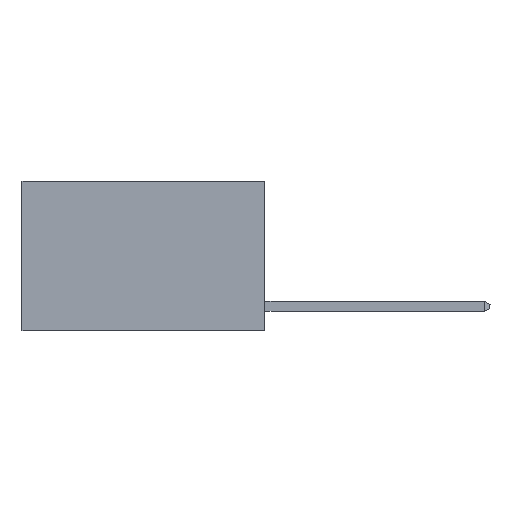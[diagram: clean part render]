
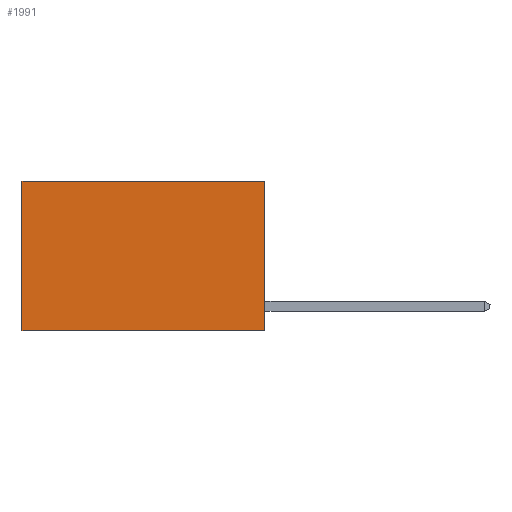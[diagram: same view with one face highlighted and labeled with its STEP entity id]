
A CAD part, left-side view. The second image highlights one B-rep face of the part: STEP entity #1991.
In plain terms, the highlighted planar face has unit normal (-1, 0, 0).
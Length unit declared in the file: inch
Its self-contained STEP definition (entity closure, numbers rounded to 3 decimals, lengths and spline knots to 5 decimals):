
#495 = VERTEX_POINT ( 'NONE', #10542 ) ;
#896 = VECTOR ( 'NONE', #9719, 39.37008 ) ;
#1484 = EDGE_CURVE ( 'NONE', #8636, #2314, #14527, .T. ) ;
#1628 = EDGE_CURVE ( 'NONE', #495, #2314, #6897, .T. ) ;
#1991 = ADVANCED_FACE ( 'NONE', ( #3237 ), #16513, .F. ) ;
#2314 = VERTEX_POINT ( 'NONE', #8777 ) ;
#2517 = DIRECTION ( 'NONE',  ( 1., 0., 0. ) ) ;
#3237 = FACE_OUTER_BOUND ( 'NONE', #6909, .T. ) ;
#3513 = CARTESIAN_POINT ( 'NONE',  ( 0.2625, 0., -0.37 ) ) ;
#3794 = ORIENTED_EDGE ( 'NONE', *, *, #1628, .T. ) ;
#4257 = ORIENTED_EDGE ( 'NONE', *, *, #1484, .F. ) ;
#4258 = EDGE_CURVE ( 'NONE', #6772, #495, #4795, .T. ) ;
#4493 = CARTESIAN_POINT ( 'NONE',  ( 0.2625, 0., 0. ) ) ;
#4739 = ORIENTED_EDGE ( 'NONE', *, *, #4258, .T. ) ;
#4795 = LINE ( 'NONE', #4493, #10032 ) ;
#5470 = VECTOR ( 'NONE', #9363, 39.37008 ) ;
#6154 = EDGE_CURVE ( 'NONE', #6772, #8636, #11171, .T. ) ;
#6772 = VERTEX_POINT ( 'NONE', #7977 ) ;
#6849 = CARTESIAN_POINT ( 'NONE',  ( 0.2625, 0.6, 0. ) ) ;
#6897 = LINE ( 'NONE', #6849, #5470 ) ;
#6909 = EDGE_LOOP ( 'NONE', ( #3794, #4257, #11476, #4739 ) ) ;
#7749 = CARTESIAN_POINT ( 'NONE',  ( 0.2625, 0., 0. ) ) ;
#7809 = CARTESIAN_POINT ( 'NONE',  ( 0.2625, 0., 0. ) ) ;
#7977 = CARTESIAN_POINT ( 'NONE',  ( 0.2625, 0., 0. ) ) ;
#8636 = VERTEX_POINT ( 'NONE', #15382 ) ;
#8777 = CARTESIAN_POINT ( 'NONE',  ( 0.2625, 0.6, -0.37 ) ) ;
#9363 = DIRECTION ( 'NONE',  ( 0., 0., -1. ) ) ;
#9719 = DIRECTION ( 'NONE',  ( 0., 1., 0. ) ) ;
#10032 = VECTOR ( 'NONE', #12118, 39.37008 ) ;
#10311 = AXIS2_PLACEMENT_3D ( 'NONE', #7749, #2517, #14184 ) ;
#10542 = CARTESIAN_POINT ( 'NONE',  ( 0.2625, 0.6, 0. ) ) ;
#11171 = LINE ( 'NONE', #7809, #13170 ) ;
#11476 = ORIENTED_EDGE ( 'NONE', *, *, #6154, .F. ) ;
#12118 = DIRECTION ( 'NONE',  ( 0., 1., 0. ) ) ;
#13170 = VECTOR ( 'NONE', #14253, 39.37008 ) ;
#14184 = DIRECTION ( 'NONE',  ( 0., 0., -1. ) ) ;
#14253 = DIRECTION ( 'NONE',  ( 0., 0., -1. ) ) ;
#14527 = LINE ( 'NONE', #3513, #896 ) ;
#15382 = CARTESIAN_POINT ( 'NONE',  ( 0.2625, 0., -0.37 ) ) ;
#16513 = PLANE ( 'NONE',  #10311 ) ;
